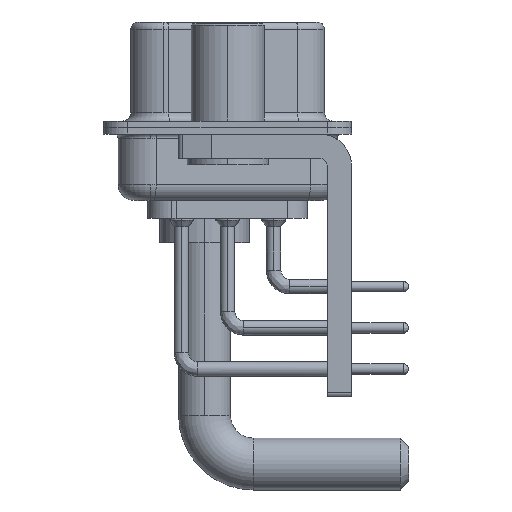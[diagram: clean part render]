
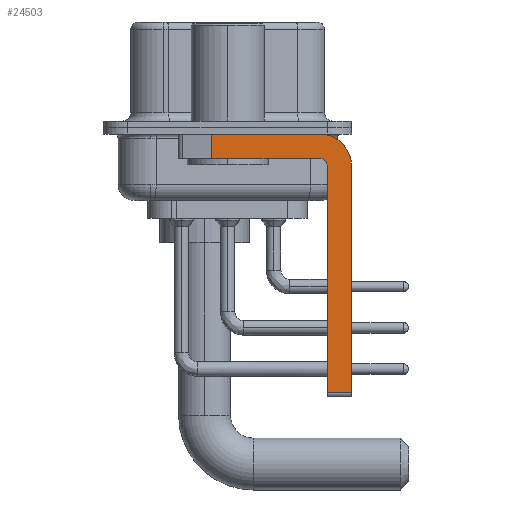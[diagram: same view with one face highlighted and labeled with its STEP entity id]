
A CAD part, left-side view. The second image highlights one B-rep face of the part: STEP entity #24503.
In plain terms, the highlighted planar face has unit normal (-1, 0, 0).
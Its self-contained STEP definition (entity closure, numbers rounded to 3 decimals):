
#77 = CARTESIAN_POINT ( 'NONE',  ( -2.9, -5.65, -2.4 ) ) ;
#1126 = EDGE_CURVE ( 'NONE', #10078, #24388, #29453, .T. ) ;
#1227 = VERTEX_POINT ( 'NONE', #17727 ) ;
#1779 = CIRCLE ( 'NONE', #29333, 0.5 ) ;
#2345 = CARTESIAN_POINT ( 'NONE',  ( -2.9, 3., -0.4 ) ) ;
#2740 = LINE ( 'NONE', #27238, #3321 ) ;
#2792 = EDGE_CURVE ( 'NONE', #24424, #10078, #1779, .T. ) ;
#3006 = CARTESIAN_POINT ( 'NONE',  ( -2.9, -5.65, -16.35 ) ) ;
#3321 = VECTOR ( 'NONE', #20395, 1000. ) ;
#4042 = CARTESIAN_POINT ( 'NONE',  ( -2.9, -5.65, -1.9 ) ) ;
#4197 = AXIS2_PLACEMENT_3D ( 'NONE', #23072, #31673, #26200 ) ;
#5576 = DIRECTION ( 'NONE',  ( 0., 0., 1. ) ) ;
#5998 = VECTOR ( 'NONE', #29873, 1000. ) ;
#6537 = EDGE_LOOP ( 'NONE', ( #19323, #28349, #24668, #13323, #25481, #11465, #20936, #24767 ) ) ;
#7496 = PLANE ( 'NONE',  #17146 ) ;
#8056 = LINE ( 'NONE', #16664, #25787 ) ;
#10078 = VERTEX_POINT ( 'NONE', #4042 ) ;
#11465 = ORIENTED_EDGE ( 'NONE', *, *, #28706, .T. ) ;
#11594 = DIRECTION ( 'NONE',  ( 0., -1., 0. ) ) ;
#13201 = CARTESIAN_POINT ( 'NONE',  ( -2.9, -6.15, -2.4 ) ) ;
#13323 = ORIENTED_EDGE ( 'NONE', *, *, #2792, .F. ) ;
#14240 = VECTOR ( 'NONE', #11594, 1000. ) ;
#14434 = CARTESIAN_POINT ( 'NONE',  ( -2.9, -6.15, -16.6 ) ) ;
#15430 = CARTESIAN_POINT ( 'NONE',  ( -2.9, 0.978, -0.4 ) ) ;
#16213 = CARTESIAN_POINT ( 'NONE',  ( -2.9, -7.65, -16.35 ) ) ;
#16664 = CARTESIAN_POINT ( 'NONE',  ( -2.9, -7.65, -2.4 ) ) ;
#16864 = DIRECTION ( 'NONE',  ( 0., 0., -1. ) ) ;
#17071 = DIRECTION ( 'NONE',  ( 0., 0., -1. ) ) ;
#17133 = DIRECTION ( 'NONE',  ( 0., 1., 0. ) ) ;
#17146 = AXIS2_PLACEMENT_3D ( 'NONE', #20196, #25694, #17071 ) ;
#17335 = DIRECTION ( 'NONE',  ( -1., 0., 0. ) ) ;
#17727 = CARTESIAN_POINT ( 'NONE',  ( -2.9, -7.65, -2.4 ) ) ;
#19323 = ORIENTED_EDGE ( 'NONE', *, *, #37970, .F. ) ;
#19816 = FACE_OUTER_BOUND ( 'NONE', #6537, .T. ) ;
#20196 = CARTESIAN_POINT ( 'NONE',  ( -2.9, -5.65, -2.4 ) ) ;
#20395 = DIRECTION ( 'NONE',  ( 0., 0., -1. ) ) ;
#20919 = EDGE_CURVE ( 'NONE', #1227, #36707, #8056, .T. ) ;
#20936 = ORIENTED_EDGE ( 'NONE', *, *, #20919, .F. ) ;
#23072 = CARTESIAN_POINT ( 'NONE',  ( -2.9, -5.65, -2.4 ) ) ;
#23520 = LINE ( 'NONE', #2345, #14240 ) ;
#24388 = VERTEX_POINT ( 'NONE', #36700 ) ;
#24424 = VERTEX_POINT ( 'NONE', #13201 ) ;
#24503 = ADVANCED_FACE ( 'NONE', ( #19816 ), #7496, .F. ) ;
#24668 = ORIENTED_EDGE ( 'NONE', *, *, #1126, .F. ) ;
#24767 = ORIENTED_EDGE ( 'NONE', *, *, #28234, .F. ) ;
#25481 = ORIENTED_EDGE ( 'NONE', *, *, #36908, .F. ) ;
#25694 = DIRECTION ( 'NONE',  ( 1., 0., 0. ) ) ;
#25787 = VECTOR ( 'NONE', #16864, 1000. ) ;
#26200 = DIRECTION ( 'NONE',  ( 0., 0., -1. ) ) ;
#26335 = CARTESIAN_POINT ( 'NONE',  ( -2.9, -5.65, -1.9 ) ) ;
#26350 = LINE ( 'NONE', #14434, #5998 ) ;
#26912 = DIRECTION ( 'NONE',  ( 0., -1., 0. ) ) ;
#27187 = VERTEX_POINT ( 'NONE', #15430 ) ;
#27238 = CARTESIAN_POINT ( 'NONE',  ( -2.9, 0.978, -1.9 ) ) ;
#28234 = EDGE_CURVE ( 'NONE', #38440, #1227, #31692, .T. ) ;
#28349 = ORIENTED_EDGE ( 'NONE', *, *, #32277, .T. ) ;
#28706 = EDGE_CURVE ( 'NONE', #30896, #36707, #32589, .T. ) ;
#29159 = CARTESIAN_POINT ( 'NONE',  ( -2.9, -6.15, -16.35 ) ) ;
#29333 = AXIS2_PLACEMENT_3D ( 'NONE', #77, #17335, #5576 ) ;
#29453 = LINE ( 'NONE', #26335, #31707 ) ;
#29723 = CARTESIAN_POINT ( 'NONE',  ( -2.9, -5.65, -0.4 ) ) ;
#29873 = DIRECTION ( 'NONE',  ( 0., 0., 1. ) ) ;
#30896 = VERTEX_POINT ( 'NONE', #29159 ) ;
#31673 = DIRECTION ( 'NONE',  ( 1., 0., 0. ) ) ;
#31692 = CIRCLE ( 'NONE', #4197, 2. ) ;
#31707 = VECTOR ( 'NONE', #17133, 1000. ) ;
#32277 = EDGE_CURVE ( 'NONE', #27187, #24388, #2740, .T. ) ;
#32589 = LINE ( 'NONE', #3006, #38623 ) ;
#36700 = CARTESIAN_POINT ( 'NONE',  ( -2.9, 0.978, -1.9 ) ) ;
#36707 = VERTEX_POINT ( 'NONE', #16213 ) ;
#36908 = EDGE_CURVE ( 'NONE', #30896, #24424, #26350, .T. ) ;
#37970 = EDGE_CURVE ( 'NONE', #27187, #38440, #23520, .T. ) ;
#38440 = VERTEX_POINT ( 'NONE', #29723 ) ;
#38623 = VECTOR ( 'NONE', #26912, 1000. ) ;
